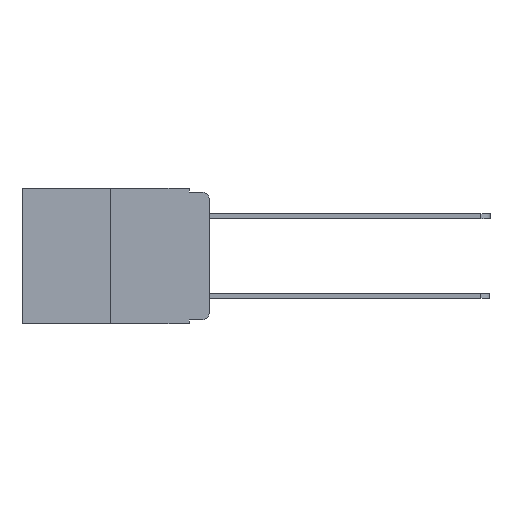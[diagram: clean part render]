
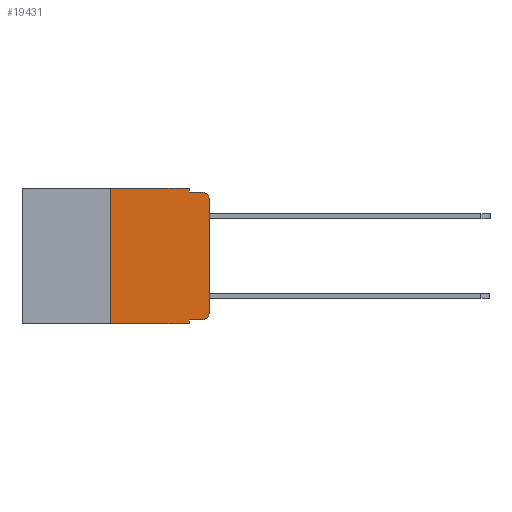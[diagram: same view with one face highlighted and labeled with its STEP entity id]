
A CAD part, left-side view. The second image highlights one B-rep face of the part: STEP entity #19431.
In plain terms, the highlighted planar face has unit normal (-1, 0, 0).
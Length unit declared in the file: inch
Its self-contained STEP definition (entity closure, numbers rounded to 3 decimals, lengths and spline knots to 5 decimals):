
#159 = LINE ( 'NONE', #10085, #8420 ) ;
#208 = LINE ( 'NONE', #13800, #9624 ) ;
#462 = CARTESIAN_POINT ( 'NONE',  ( 0., 0.051, 0. ) ) ;
#879 = CIRCLE ( 'NONE', #2121, 0.02 ) ;
#1018 = VECTOR ( 'NONE', #15106, 39.37008 ) ;
#1531 = DIRECTION ( 'NONE',  ( 0., 0., -1. ) ) ;
#2121 = AXIS2_PLACEMENT_3D ( 'NONE', #17951, #7090, #19712 ) ;
#2402 = VECTOR ( 'NONE', #16529, 39.37008 ) ;
#3228 = VECTOR ( 'NONE', #21085, 39.37008 ) ;
#4115 = CARTESIAN_POINT ( 'NONE',  ( 0., 0.02, -0.333 ) ) ;
#4213 = VERTEX_POINT ( 'NONE', #19763 ) ;
#4684 = DIRECTION ( 'NONE',  ( 0., 0., 1. ) ) ;
#4723 = ORIENTED_EDGE ( 'NONE', *, *, #20269, .T. ) ;
#4853 = ORIENTED_EDGE ( 'NONE', *, *, #13630, .T. ) ;
#5062 = ORIENTED_EDGE ( 'NONE', *, *, #8390, .F. ) ;
#5470 = ORIENTED_EDGE ( 'NONE', *, *, #6373, .F. ) ;
#5630 = ORIENTED_EDGE ( 'NONE', *, *, #15880, .F. ) ;
#5931 = ORIENTED_EDGE ( 'NONE', *, *, #21877, .F. ) ;
#6255 = ORIENTED_EDGE ( 'NONE', *, *, #21284, .T. ) ;
#6373 = EDGE_CURVE ( 'NONE', #17578, #22011, #11679, .T. ) ;
#6454 = CARTESIAN_POINT ( 'NONE',  ( 0., 0.051, 0. ) ) ;
#6651 = LINE ( 'NONE', #13299, #1018 ) ;
#6661 = ORIENTED_EDGE ( 'NONE', *, *, #18350, .F. ) ;
#6796 = ORIENTED_EDGE ( 'NONE', *, *, #17903, .T. ) ;
#6958 = CARTESIAN_POINT ( 'NONE',  ( 0., 0., -0.03 ) ) ;
#6989 = ORIENTED_EDGE ( 'NONE', *, *, #10663, .T. ) ;
#7090 = DIRECTION ( 'NONE',  ( -1., 0., 0. ) ) ;
#7239 = DIRECTION ( 'NONE',  ( 0., 0., -1. ) ) ;
#7506 = VERTEX_POINT ( 'NONE', #9886 ) ;
#7574 = CARTESIAN_POINT ( 'NONE',  ( 0., 0.051, -0.01 ) ) ;
#7732 = VERTEX_POINT ( 'NONE', #10575 ) ;
#8250 = VERTEX_POINT ( 'NONE', #19715 ) ;
#8390 = EDGE_CURVE ( 'NONE', #22011, #8250, #8454, .T. ) ;
#8420 = VECTOR ( 'NONE', #11918, 39.37008 ) ;
#8454 = LINE ( 'NONE', #7574, #12751 ) ;
#8530 = CARTESIAN_POINT ( 'NONE',  ( 0., 0.473, -0.343 ) ) ;
#9624 = VECTOR ( 'NONE', #4684, 39.37008 ) ;
#9850 = VECTOR ( 'NONE', #21460, 39.37008 ) ;
#9886 = CARTESIAN_POINT ( 'NONE',  ( 0., 0.25, 0. ) ) ;
#10085 = CARTESIAN_POINT ( 'NONE',  ( 0., 0.473, 0. ) ) ;
#10575 = CARTESIAN_POINT ( 'NONE',  ( 0., 0., -0.313 ) ) ;
#10663 = EDGE_CURVE ( 'NONE', #21710, #7732, #15205, .T. ) ;
#10770 = PLANE ( 'NONE',  #16700 ) ;
#10848 = CARTESIAN_POINT ( 'NONE',  ( 0., 0.473, 0. ) ) ;
#11086 = VERTEX_POINT ( 'NONE', #6958 ) ;
#11679 = LINE ( 'NONE', #6454, #12240 ) ;
#11918 = DIRECTION ( 'NONE',  ( 0., -1., 0. ) ) ;
#12240 = VECTOR ( 'NONE', #19120, 39.37008 ) ;
#12420 = CARTESIAN_POINT ( 'NONE',  ( 0., 0.051, -0.01 ) ) ;
#12693 = DIRECTION ( 'NONE',  ( -1., 0., 0. ) ) ;
#12751 = VECTOR ( 'NONE', #20181, 39.37008 ) ;
#13299 = CARTESIAN_POINT ( 'NONE',  ( 0., 0.051, 0. ) ) ;
#13608 = VERTEX_POINT ( 'NONE', #19558 ) ;
#13630 = EDGE_CURVE ( 'NONE', #11086, #8250, #879, .T. ) ;
#13674 = LINE ( 'NONE', #8530, #3228 ) ;
#13800 = CARTESIAN_POINT ( 'NONE',  ( 0., 0.25, 0. ) ) ;
#14064 = VERTEX_POINT ( 'NONE', #22458 ) ;
#14335 = FACE_OUTER_BOUND ( 'NONE', #20743, .T. ) ;
#14741 = CARTESIAN_POINT ( 'NONE',  ( 0., 0., 0. ) ) ;
#15106 = DIRECTION ( 'NONE',  ( 0., 0., -1. ) ) ;
#15205 = CIRCLE ( 'NONE', #17766, 0.02 ) ;
#15880 = EDGE_CURVE ( 'NONE', #7506, #17578, #159, .T. ) ;
#16529 = DIRECTION ( 'NONE',  ( 0., 0., 1. ) ) ;
#16700 = AXIS2_PLACEMENT_3D ( 'NONE', #10848, #18092, #7239 ) ;
#17578 = VERTEX_POINT ( 'NONE', #462 ) ;
#17766 = AXIS2_PLACEMENT_3D ( 'NONE', #23232, #12693, #1531 ) ;
#17903 = EDGE_CURVE ( 'NONE', #13608, #21710, #19398, .T. ) ;
#17951 = CARTESIAN_POINT ( 'NONE',  ( 0., 0.02, -0.03 ) ) ;
#18092 = DIRECTION ( 'NONE',  ( 1., 0., 0. ) ) ;
#18350 = EDGE_CURVE ( 'NONE', #13608, #14064, #6651, .T. ) ;
#19120 = DIRECTION ( 'NONE',  ( 0., 0., -1. ) ) ;
#19398 = LINE ( 'NONE', #19754, #9850 ) ;
#19431 = ADVANCED_FACE ( 'NONE', ( #14335 ), #10770, .F. ) ;
#19558 = CARTESIAN_POINT ( 'NONE',  ( 0., 0.051, -0.333 ) ) ;
#19712 = DIRECTION ( 'NONE',  ( 0., 0., -1. ) ) ;
#19715 = CARTESIAN_POINT ( 'NONE',  ( 0., 0.02, -0.01 ) ) ;
#19754 = CARTESIAN_POINT ( 'NONE',  ( 0., 0.051, -0.333 ) ) ;
#19763 = CARTESIAN_POINT ( 'NONE',  ( 0., 0.25, -0.343 ) ) ;
#20181 = DIRECTION ( 'NONE',  ( 0., -1., 0. ) ) ;
#20269 = EDGE_CURVE ( 'NONE', #7732, #11086, #21194, .T. ) ;
#20743 = EDGE_LOOP ( 'NONE', ( #4723, #4853, #5062, #5470, #5630, #5931, #6255, #6661, #6796, #6989 ) ) ;
#21085 = DIRECTION ( 'NONE',  ( 0., -1., 0. ) ) ;
#21194 = LINE ( 'NONE', #14741, #2402 ) ;
#21284 = EDGE_CURVE ( 'NONE', #4213, #14064, #13674, .T. ) ;
#21460 = DIRECTION ( 'NONE',  ( 0., -1., 0. ) ) ;
#21710 = VERTEX_POINT ( 'NONE', #4115 ) ;
#21877 = EDGE_CURVE ( 'NONE', #4213, #7506, #208, .T. ) ;
#22011 = VERTEX_POINT ( 'NONE', #12420 ) ;
#22458 = CARTESIAN_POINT ( 'NONE',  ( 0., 0.051, -0.343 ) ) ;
#23232 = CARTESIAN_POINT ( 'NONE',  ( 0., 0.02, -0.313 ) ) ;
